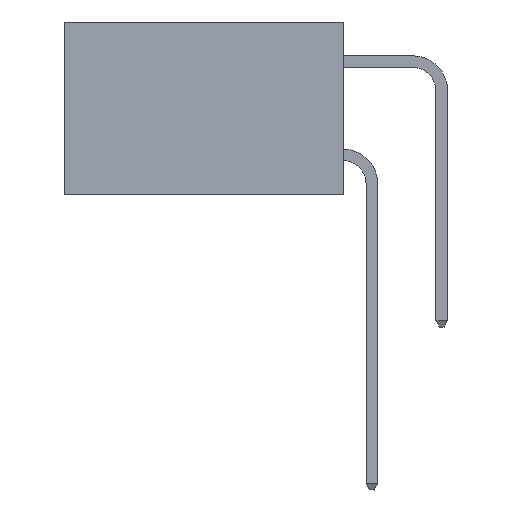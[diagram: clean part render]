
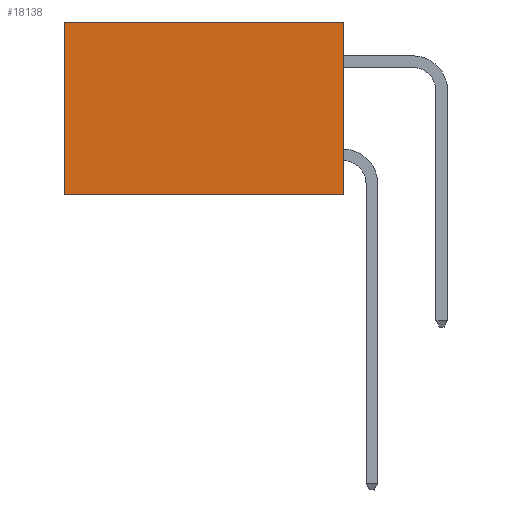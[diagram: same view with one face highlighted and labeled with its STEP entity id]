
A CAD part, left-side view. The second image highlights one B-rep face of the part: STEP entity #18138.
In plain terms, the highlighted planar face has unit normal (-1, 0, 0).
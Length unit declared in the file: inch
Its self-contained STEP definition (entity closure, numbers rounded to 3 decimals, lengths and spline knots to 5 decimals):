
#662 = AXIS2_PLACEMENT_3D ( 'NONE', #7288, #20433, #9196 ) ;
#784 = LINE ( 'NONE', #10244, #14089 ) ;
#986 = VERTEX_POINT ( 'NONE', #19324 ) ;
#999 = EDGE_CURVE ( 'NONE', #986, #12352, #24025, .T. ) ;
#1161 = DIRECTION ( 'NONE',  ( 0., 1., 0. ) ) ;
#1418 = DIRECTION ( 'NONE',  ( 0., 0., -1. ) ) ;
#1914 = FACE_OUTER_BOUND ( 'NONE', #5933, .T. ) ;
#3025 = CARTESIAN_POINT ( 'NONE',  ( 0.298, 0., 0. ) ) ;
#3999 = EDGE_CURVE ( 'NONE', #10227, #12352, #784, .T. ) ;
#5407 = PLANE ( 'NONE',  #662 ) ;
#5933 = EDGE_LOOP ( 'NONE', ( #18169, #15081, #12824, #12116 ) ) ;
#6676 = VECTOR ( 'NONE', #1161, 39.37008 ) ;
#7288 = CARTESIAN_POINT ( 'NONE',  ( 0.298, 0., 0. ) ) ;
#9196 = DIRECTION ( 'NONE',  ( 0., 0., -1. ) ) ;
#10227 = VERTEX_POINT ( 'NONE', #23498 ) ;
#10244 = CARTESIAN_POINT ( 'NONE',  ( 0.298, 0., -0.37 ) ) ;
#10602 = DIRECTION ( 'NONE',  ( 0., 0., -1. ) ) ;
#11768 = DIRECTION ( 'NONE',  ( 0., 1., 0. ) ) ;
#12116 = ORIENTED_EDGE ( 'NONE', *, *, #21969, .T. ) ;
#12352 = VERTEX_POINT ( 'NONE', #15543 ) ;
#12824 = ORIENTED_EDGE ( 'NONE', *, *, #24242, .F. ) ;
#12912 = VECTOR ( 'NONE', #1418, 39.37008 ) ;
#14089 = VECTOR ( 'NONE', #11768, 39.37008 ) ;
#15081 = ORIENTED_EDGE ( 'NONE', *, *, #3999, .F. ) ;
#15102 = VERTEX_POINT ( 'NONE', #22402 ) ;
#15543 = CARTESIAN_POINT ( 'NONE',  ( 0.298, 0.6, -0.37 ) ) ;
#16167 = CARTESIAN_POINT ( 'NONE',  ( 0.298, 0., 0. ) ) ;
#18138 = ADVANCED_FACE ( 'NONE', ( #1914 ), #5407, .F. ) ;
#18169 = ORIENTED_EDGE ( 'NONE', *, *, #999, .T. ) ;
#18944 = VECTOR ( 'NONE', #10602, 39.37008 ) ;
#19324 = CARTESIAN_POINT ( 'NONE',  ( 0.298, 0.6, 0. ) ) ;
#19361 = CARTESIAN_POINT ( 'NONE',  ( 0.298, 0.6, 0. ) ) ;
#20433 = DIRECTION ( 'NONE',  ( 1., 0., 0. ) ) ;
#21679 = LINE ( 'NONE', #3025, #6676 ) ;
#21969 = EDGE_CURVE ( 'NONE', #15102, #986, #21679, .T. ) ;
#22402 = CARTESIAN_POINT ( 'NONE',  ( 0.298, 0., 0. ) ) ;
#23498 = CARTESIAN_POINT ( 'NONE',  ( 0.298, 0., -0.37 ) ) ;
#23899 = LINE ( 'NONE', #16167, #18944 ) ;
#24025 = LINE ( 'NONE', #19361, #12912 ) ;
#24242 = EDGE_CURVE ( 'NONE', #15102, #10227, #23899, .T. ) ;
